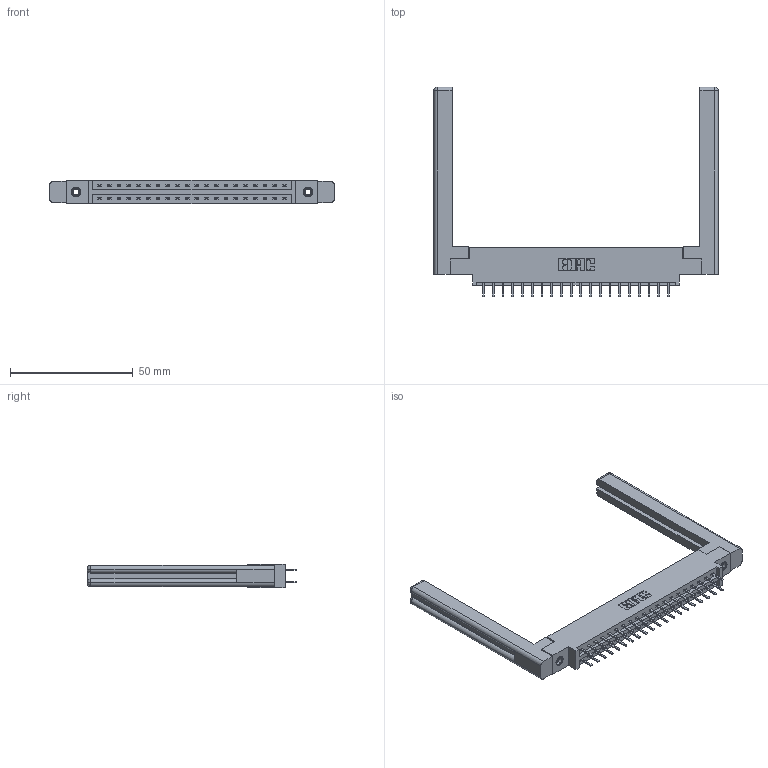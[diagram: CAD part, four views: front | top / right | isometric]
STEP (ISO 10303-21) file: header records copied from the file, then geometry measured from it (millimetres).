
FILE_DESCRIPTION (( 'STEP AP203' ), '1' );
FILE_NAME ('387-040-520-858.STEP', '2019-10-17T23:02:22', ( '' ), ( '' ), 'SwSTEP 2.0', 'SolidWorks 2016', '' );
FILE_SCHEMA (( 'CONFIG_CONTROL_DESIGN' ));
Length unit declared in the file: inch
Products named in the file (5): 307-220-058; 345-250-001_345-250-001-102; 345-292-001_345-293-120; 337 Part_0.170 Offset - 0.156 Dia-TI; 387-040-520-858
Assembly tree (45 placements, depth 2):
  387-040-520-858
    337 Part_0.170 Offset - 0.156 Dia-TI
    345-292-001_345-293-120  x40
    345-250-001_345-250-001-102  x2
    307-220-058  x2
Bounding box: 115.87 x 85.43 x 9.4 mm (x, y, z)
Volume: 18926.2 mm3; surface area: 18212.4 mm2
Topology: 45 solids, 45 shells, 2580 faces, 7437 edges, 4838 vertices
Faces by surface type: plane 1758, cylinder 798, cone 12, torus 12
Entity records: 21232 total; most frequent: CARTESIAN_POINT 3617, ORIENTED_EDGE 3480, DIRECTION 3120, EDGE_CURVE 1740, VECTOR 1560, LINE 1560, VERTEX_POINT 1150, AXIS2_PLACEMENT_3D 780
